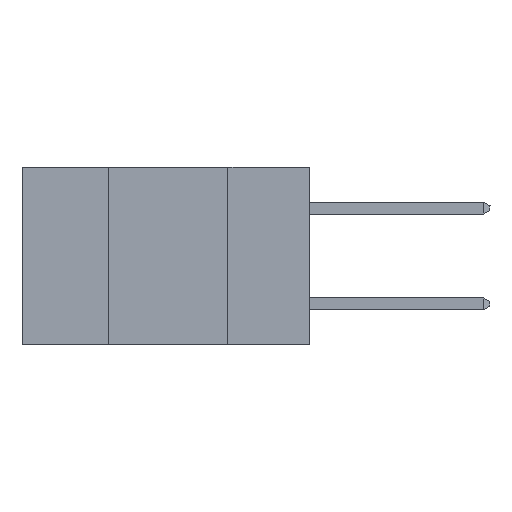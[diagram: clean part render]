
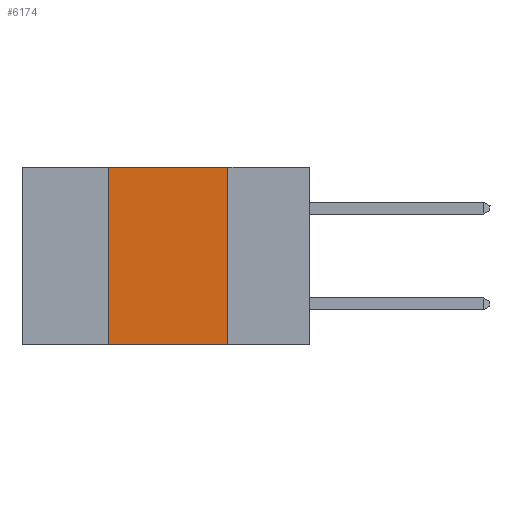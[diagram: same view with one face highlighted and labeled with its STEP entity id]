
A CAD part, left-side view. The second image highlights one B-rep face of the part: STEP entity #6174.
In plain terms, the highlighted planar face has unit normal (-1, 0, 0).
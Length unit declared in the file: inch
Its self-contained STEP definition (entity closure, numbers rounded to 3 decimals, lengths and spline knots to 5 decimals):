
#221 = EDGE_LOOP ( 'NONE', ( #27586, #4575, #6012, #10459 ) ) ;
#659 = CARTESIAN_POINT ( 'NONE',  ( 0., 0.6, 0. ) ) ;
#881 = CARTESIAN_POINT ( 'NONE',  ( 0., 0.17, 0. ) ) ;
#2484 = VERTEX_POINT ( 'NONE', #11617 ) ;
#2788 = VECTOR ( 'NONE', #14109, 39.37008 ) ;
#3120 = DIRECTION ( 'NONE',  ( 0., 0., -1. ) ) ;
#4246 = CARTESIAN_POINT ( 'NONE',  ( 0., 0.42, 0. ) ) ;
#4575 = ORIENTED_EDGE ( 'NONE', *, *, #23987, .F. ) ;
#5963 = AXIS2_PLACEMENT_3D ( 'NONE', #20580, #20221, #3120 ) ;
#6012 = ORIENTED_EDGE ( 'NONE', *, *, #11584, .F. ) ;
#6174 = ADVANCED_FACE ( 'NONE', ( #9821 ), #26129, .F. ) ;
#8279 = EDGE_CURVE ( 'NONE', #2484, #10030, #9121, .T. ) ;
#9121 = LINE ( 'NONE', #881, #2788 ) ;
#9821 = FACE_OUTER_BOUND ( 'NONE', #221, .T. ) ;
#10030 = VERTEX_POINT ( 'NONE', #12074 ) ;
#10190 = LINE ( 'NONE', #33023, #17462 ) ;
#10459 = ORIENTED_EDGE ( 'NONE', *, *, #31234, .T. ) ;
#11584 = EDGE_CURVE ( 'NONE', #35318, #30492, #36255, .T. ) ;
#11617 = CARTESIAN_POINT ( 'NONE',  ( 0., 0.17, 0. ) ) ;
#12074 = CARTESIAN_POINT ( 'NONE',  ( 0., 0.17, -0.37 ) ) ;
#13272 = DIRECTION ( 'NONE',  ( 0., 0., 1. ) ) ;
#14109 = DIRECTION ( 'NONE',  ( 0., 0., -1. ) ) ;
#15858 = DIRECTION ( 'NONE',  ( 0., -1., 0. ) ) ;
#16055 = DIRECTION ( 'NONE',  ( 0., -1., 0. ) ) ;
#17462 = VECTOR ( 'NONE', #15858, 39.37008 ) ;
#18363 = LINE ( 'NONE', #659, #32001 ) ;
#18544 = CARTESIAN_POINT ( 'NONE',  ( 0., 0.42, 0. ) ) ;
#20221 = DIRECTION ( 'NONE',  ( 1., 0., 0. ) ) ;
#20580 = CARTESIAN_POINT ( 'NONE',  ( 0., 0.6, 0. ) ) ;
#22490 = CARTESIAN_POINT ( 'NONE',  ( 0., 0.42, -0.37 ) ) ;
#23987 = EDGE_CURVE ( 'NONE', #30492, #2484, #18363, .T. ) ;
#26129 = PLANE ( 'NONE',  #5963 ) ;
#27586 = ORIENTED_EDGE ( 'NONE', *, *, #8279, .F. ) ;
#30492 = VERTEX_POINT ( 'NONE', #18544 ) ;
#31234 = EDGE_CURVE ( 'NONE', #35318, #10030, #10190, .T. ) ;
#32001 = VECTOR ( 'NONE', #16055, 39.37008 ) ;
#33023 = CARTESIAN_POINT ( 'NONE',  ( 0., 0.6, -0.37 ) ) ;
#34884 = VECTOR ( 'NONE', #13272, 39.37008 ) ;
#35318 = VERTEX_POINT ( 'NONE', #22490 ) ;
#36255 = LINE ( 'NONE', #4246, #34884 ) ;
